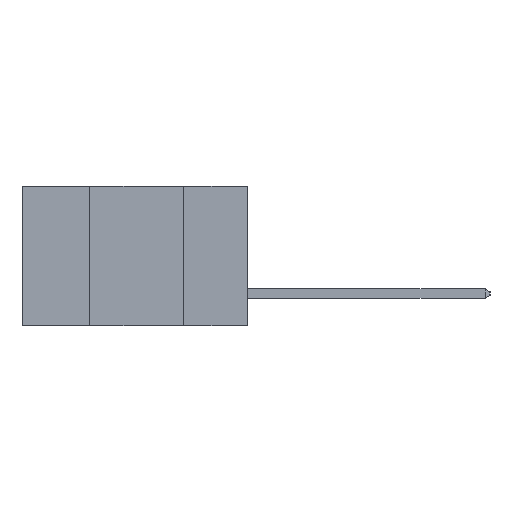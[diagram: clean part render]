
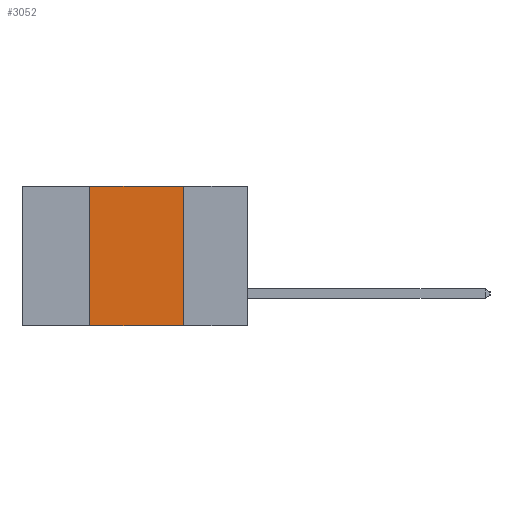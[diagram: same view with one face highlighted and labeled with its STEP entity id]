
A CAD part, left-side view. The second image highlights one B-rep face of the part: STEP entity #3052.
In plain terms, the highlighted planar face has unit normal (-1, 0, 0).
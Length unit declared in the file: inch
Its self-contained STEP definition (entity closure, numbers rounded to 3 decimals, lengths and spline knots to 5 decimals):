
#47 = CARTESIAN_POINT ( 'NONE',  ( 0., 0.6, -0.37 ) ) ;
#666 = VERTEX_POINT ( 'NONE', #10688 ) ;
#1115 = DIRECTION ( 'NONE',  ( 0., 0., -1. ) ) ;
#2435 = ORIENTED_EDGE ( 'NONE', *, *, #2450, .F. ) ;
#2450 = EDGE_CURVE ( 'NONE', #5242, #666, #22391, .T. ) ;
#3052 = ADVANCED_FACE ( 'NONE', ( #23850 ), #3365, .F. ) ;
#3289 = VERTEX_POINT ( 'NONE', #24344 ) ;
#3365 = PLANE ( 'NONE',  #20329 ) ;
#5242 = VERTEX_POINT ( 'NONE', #20607 ) ;
#6880 = DIRECTION ( 'NONE',  ( 0., 0., 1. ) ) ;
#7477 = CARTESIAN_POINT ( 'NONE',  ( 0., 0.17, 0. ) ) ;
#7724 = EDGE_CURVE ( 'NONE', #3289, #22036, #13311, .T. ) ;
#8357 = VECTOR ( 'NONE', #9447, 39.37008 ) ;
#8851 = ORIENTED_EDGE ( 'NONE', *, *, #18788, .F. ) ;
#9447 = DIRECTION ( 'NONE',  ( 0., 0., -1. ) ) ;
#9775 = DIRECTION ( 'NONE',  ( 0., -1., 0. ) ) ;
#10393 = ORIENTED_EDGE ( 'NONE', *, *, #18973, .F. ) ;
#10688 = CARTESIAN_POINT ( 'NONE',  ( 0., 0.17, 0. ) ) ;
#11521 = CARTESIAN_POINT ( 'NONE',  ( 0., 0.17, -0.37 ) ) ;
#12717 = CARTESIAN_POINT ( 'NONE',  ( 0., 0.42, 0. ) ) ;
#13233 = VECTOR ( 'NONE', #6880, 39.37008 ) ;
#13311 = LINE ( 'NONE', #47, #17922 ) ;
#13527 = LINE ( 'NONE', #7477, #8357 ) ;
#13541 = DIRECTION ( 'NONE',  ( 0., -1., 0. ) ) ;
#14317 = CARTESIAN_POINT ( 'NONE',  ( 0., 0.6, 0. ) ) ;
#17220 = VECTOR ( 'NONE', #13541, 39.37008 ) ;
#17515 = CARTESIAN_POINT ( 'NONE',  ( 0., 0.6, 0. ) ) ;
#17922 = VECTOR ( 'NONE', #9775, 39.37008 ) ;
#18788 = EDGE_CURVE ( 'NONE', #3289, #5242, #23040, .T. ) ;
#18973 = EDGE_CURVE ( 'NONE', #666, #22036, #13527, .T. ) ;
#20329 = AXIS2_PLACEMENT_3D ( 'NONE', #17515, #20583, #1115 ) ;
#20583 = DIRECTION ( 'NONE',  ( 1., 0., 0. ) ) ;
#20607 = CARTESIAN_POINT ( 'NONE',  ( 0., 0.42, 0. ) ) ;
#21820 = ORIENTED_EDGE ( 'NONE', *, *, #7724, .T. ) ;
#22036 = VERTEX_POINT ( 'NONE', #11521 ) ;
#22391 = LINE ( 'NONE', #14317, #17220 ) ;
#22433 = EDGE_LOOP ( 'NONE', ( #10393, #2435, #8851, #21820 ) ) ;
#23040 = LINE ( 'NONE', #12717, #13233 ) ;
#23850 = FACE_OUTER_BOUND ( 'NONE', #22433, .T. ) ;
#24344 = CARTESIAN_POINT ( 'NONE',  ( 0., 0.42, -0.37 ) ) ;
